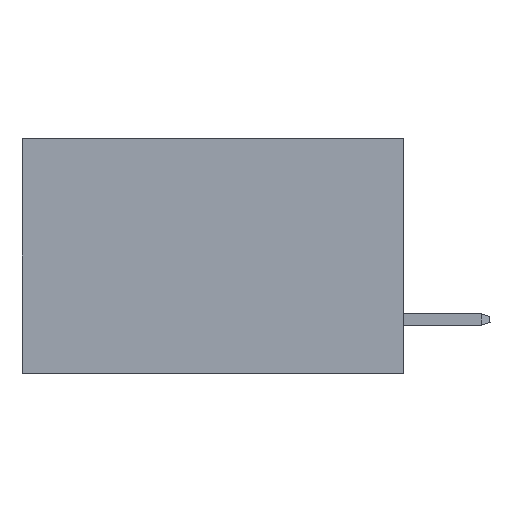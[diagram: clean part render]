
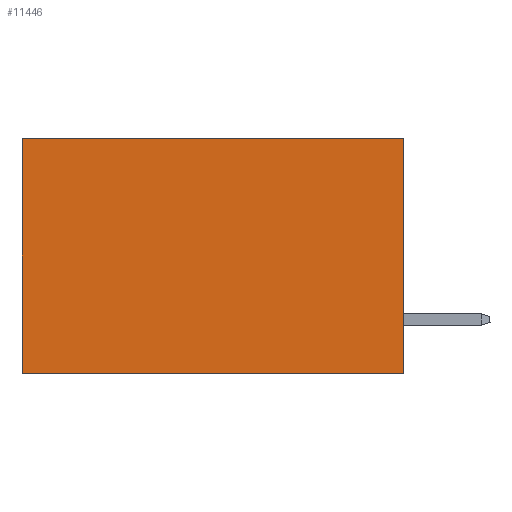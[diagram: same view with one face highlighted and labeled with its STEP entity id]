
A CAD part, left-side view. The second image highlights one B-rep face of the part: STEP entity #11446.
In plain terms, the highlighted planar face has unit normal (-1, 0, 0).
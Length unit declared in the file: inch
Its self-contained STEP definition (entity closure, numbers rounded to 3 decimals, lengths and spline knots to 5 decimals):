
#843 = CARTESIAN_POINT ( 'NONE',  ( 0.2875, 0., 0. ) ) ;
#2791 = CARTESIAN_POINT ( 'NONE',  ( 0.2875, 0.6, 0. ) ) ;
#3190 = EDGE_CURVE ( 'NONE', #23392, #12512, #21030, .T. ) ;
#3818 = AXIS2_PLACEMENT_3D ( 'NONE', #10087, #20961, #26137 ) ;
#5163 = DIRECTION ( 'NONE',  ( 0., 0., -1. ) ) ;
#6588 = CARTESIAN_POINT ( 'NONE',  ( 0.2875, 0., 0. ) ) ;
#8962 = EDGE_CURVE ( 'NONE', #17936, #23392, #21311, .T. ) ;
#9936 = ORIENTED_EDGE ( 'NONE', *, *, #13269, .T. ) ;
#10087 = CARTESIAN_POINT ( 'NONE',  ( 0.2875, 0., 0. ) ) ;
#11165 = VECTOR ( 'NONE', #18692, 39.37008 ) ;
#11273 = VERTEX_POINT ( 'NONE', #30560 ) ;
#11356 = EDGE_CURVE ( 'NONE', #17936, #11273, #33243, .T. ) ;
#11446 = ADVANCED_FACE ( 'NONE', ( #28764 ), #34461, .F. ) ;
#12512 = VERTEX_POINT ( 'NONE', #29891 ) ;
#12573 = CARTESIAN_POINT ( 'NONE',  ( 0.2875, 0., -0.37 ) ) ;
#12777 = ORIENTED_EDGE ( 'NONE', *, *, #3190, .F. ) ;
#13269 = EDGE_CURVE ( 'NONE', #11273, #12512, #27143, .T. ) ;
#13579 = DIRECTION ( 'NONE',  ( 0., 0., -1. ) ) ;
#15810 = VECTOR ( 'NONE', #13579, 39.37008 ) ;
#16747 = VECTOR ( 'NONE', #5163, 39.37008 ) ;
#17936 = VERTEX_POINT ( 'NONE', #843 ) ;
#18692 = DIRECTION ( 'NONE',  ( 0., 1., 0. ) ) ;
#20961 = DIRECTION ( 'NONE',  ( 1., 0., 0. ) ) ;
#21027 = ORIENTED_EDGE ( 'NONE', *, *, #8962, .F. ) ;
#21030 = LINE ( 'NONE', #27259, #11165 ) ;
#21311 = LINE ( 'NONE', #32146, #16747 ) ;
#23392 = VERTEX_POINT ( 'NONE', #12573 ) ;
#25368 = VECTOR ( 'NONE', #27906, 39.37008 ) ;
#26137 = DIRECTION ( 'NONE',  ( 0., 0., -1. ) ) ;
#27143 = LINE ( 'NONE', #2791, #15810 ) ;
#27259 = CARTESIAN_POINT ( 'NONE',  ( 0.2875, 0., -0.37 ) ) ;
#27906 = DIRECTION ( 'NONE',  ( 0., 1., 0. ) ) ;
#28764 = FACE_OUTER_BOUND ( 'NONE', #29046, .T. ) ;
#29046 = EDGE_LOOP ( 'NONE', ( #9936, #12777, #21027, #30149 ) ) ;
#29891 = CARTESIAN_POINT ( 'NONE',  ( 0.2875, 0.6, -0.37 ) ) ;
#30149 = ORIENTED_EDGE ( 'NONE', *, *, #11356, .T. ) ;
#30560 = CARTESIAN_POINT ( 'NONE',  ( 0.2875, 0.6, 0. ) ) ;
#32146 = CARTESIAN_POINT ( 'NONE',  ( 0.2875, 0., 0. ) ) ;
#33243 = LINE ( 'NONE', #6588, #25368 ) ;
#34461 = PLANE ( 'NONE',  #3818 ) ;
